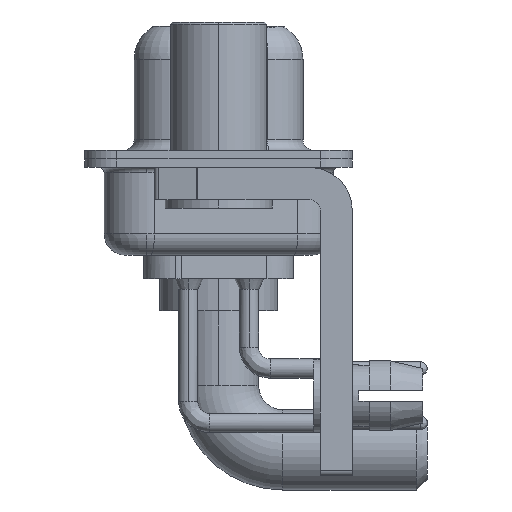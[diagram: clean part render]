
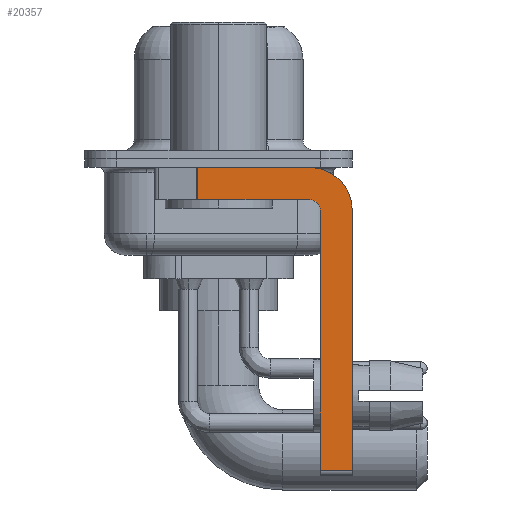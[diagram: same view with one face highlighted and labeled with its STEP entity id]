
A CAD part, left-side view. The second image highlights one B-rep face of the part: STEP entity #20357.
In plain terms, the highlighted planar face has unit normal (-1, 0, 0).
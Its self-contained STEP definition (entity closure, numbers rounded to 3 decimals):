
#67 = DIRECTION ( 'NONE',  ( 0., 1., 0. ) ) ;
#75 = CARTESIAN_POINT ( 'NONE',  ( -2.9, -4.25, -0.4 ) ) ;
#458 = EDGE_CURVE ( 'NONE', #22829, #11674, #7403, .T. ) ;
#1212 = CARTESIAN_POINT ( 'NONE',  ( -2.9, -6.25, -14.55 ) ) ;
#1302 = DIRECTION ( 'NONE',  ( 0., 0., -1. ) ) ;
#1585 = CARTESIAN_POINT ( 'NONE',  ( -2.9, -4.25, -2.4 ) ) ;
#1908 = VERTEX_POINT ( 'NONE', #1212 ) ;
#1944 = AXIS2_PLACEMENT_3D ( 'NONE', #1585, #7960, #22071 ) ;
#2185 = ORIENTED_EDGE ( 'NONE', *, *, #17712, .F. ) ;
#2240 = VERTEX_POINT ( 'NONE', #11292 ) ;
#2496 = CARTESIAN_POINT ( 'NONE',  ( -2.9, -6.25, -2.4 ) ) ;
#2915 = LINE ( 'NONE', #19490, #25348 ) ;
#3138 = VECTOR ( 'NONE', #67, 1000. ) ;
#3309 = DIRECTION ( 'NONE',  ( 0., 0., 1. ) ) ;
#4119 = CARTESIAN_POINT ( 'NONE',  ( -2.9, -4.25, -1.9 ) ) ;
#4531 = CARTESIAN_POINT ( 'NONE',  ( -2.9, -4.25, -2.4 ) ) ;
#4734 = FACE_OUTER_BOUND ( 'NONE', #25902, .T. ) ;
#5953 = ORIENTED_EDGE ( 'NONE', *, *, #12945, .T. ) ;
#6385 = VECTOR ( 'NONE', #1302, 1000. ) ;
#6635 = PLANE ( 'NONE',  #25608 ) ;
#7281 = CARTESIAN_POINT ( 'NONE',  ( -2.9, 0.978, -1.9 ) ) ;
#7403 = LINE ( 'NONE', #7281, #6385 ) ;
#7960 = DIRECTION ( 'NONE',  ( -1., 0., 0. ) ) ;
#8076 = LINE ( 'NONE', #19209, #13246 ) ;
#8776 = VERTEX_POINT ( 'NONE', #75 ) ;
#8987 = DIRECTION ( 'NONE',  ( 0., -1., 0. ) ) ;
#9568 = CARTESIAN_POINT ( 'NONE',  ( -2.9, 3., -0.4 ) ) ;
#10225 = VECTOR ( 'NONE', #20009, 1000. ) ;
#10948 = VERTEX_POINT ( 'NONE', #14437 ) ;
#11292 = CARTESIAN_POINT ( 'NONE',  ( -2.9, -4.75, -2.4 ) ) ;
#11674 = VERTEX_POINT ( 'NONE', #16979 ) ;
#11741 = LINE ( 'NONE', #9568, #10225 ) ;
#12421 = VERTEX_POINT ( 'NONE', #2496 ) ;
#12475 = CARTESIAN_POINT ( 'NONE',  ( -2.9, -4.25, -1.9 ) ) ;
#12802 = ORIENTED_EDGE ( 'NONE', *, *, #15644, .F. ) ;
#12945 = EDGE_CURVE ( 'NONE', #10948, #1908, #13219, .T. ) ;
#13051 = DIRECTION ( 'NONE',  ( 1., 0., 0. ) ) ;
#13219 = LINE ( 'NONE', #17435, #19891 ) ;
#13246 = VECTOR ( 'NONE', #24734, 1000. ) ;
#14437 = CARTESIAN_POINT ( 'NONE',  ( -2.9, -4.75, -14.55 ) ) ;
#14476 = LINE ( 'NONE', #4119, #3138 ) ;
#14824 = DIRECTION ( 'NONE',  ( 0., 0., -1. ) ) ;
#15644 = EDGE_CURVE ( 'NONE', #8776, #12421, #19301, .T. ) ;
#16699 = ORIENTED_EDGE ( 'NONE', *, *, #25475, .F. ) ;
#16734 = EDGE_CURVE ( 'NONE', #2240, #23734, #17162, .T. ) ;
#16979 = CARTESIAN_POINT ( 'NONE',  ( -2.9, 0.978, -1.9 ) ) ;
#17141 = EDGE_CURVE ( 'NONE', #10948, #2240, #2915, .T. ) ;
#17162 = CIRCLE ( 'NONE', #1944, 0.5 ) ;
#17435 = CARTESIAN_POINT ( 'NONE',  ( -2.9, -4.25, -14.55 ) ) ;
#17712 = EDGE_CURVE ( 'NONE', #22829, #8776, #11741, .T. ) ;
#18380 = AXIS2_PLACEMENT_3D ( 'NONE', #4531, #19078, #19330 ) ;
#19078 = DIRECTION ( 'NONE',  ( 1., 0., 0. ) ) ;
#19209 = CARTESIAN_POINT ( 'NONE',  ( -2.9, -6.25, -2.4 ) ) ;
#19301 = CIRCLE ( 'NONE', #18380, 2. ) ;
#19330 = DIRECTION ( 'NONE',  ( 0., 0., -1. ) ) ;
#19490 = CARTESIAN_POINT ( 'NONE',  ( -2.9, -4.75, -14.8 ) ) ;
#19891 = VECTOR ( 'NONE', #8987, 1000. ) ;
#20009 = DIRECTION ( 'NONE',  ( 0., -1., 0. ) ) ;
#20357 = ADVANCED_FACE ( 'NONE', ( #4734 ), #6635, .F. ) ;
#21530 = ORIENTED_EDGE ( 'NONE', *, *, #16734, .F. ) ;
#22055 = ORIENTED_EDGE ( 'NONE', *, *, #17141, .F. ) ;
#22071 = DIRECTION ( 'NONE',  ( 0., 0., 1. ) ) ;
#22095 = ORIENTED_EDGE ( 'NONE', *, *, #22131, .F. ) ;
#22131 = EDGE_CURVE ( 'NONE', #23734, #11674, #14476, .T. ) ;
#22774 = CARTESIAN_POINT ( 'NONE',  ( -2.9, -4.25, -2.4 ) ) ;
#22788 = ORIENTED_EDGE ( 'NONE', *, *, #458, .T. ) ;
#22829 = VERTEX_POINT ( 'NONE', #25909 ) ;
#23734 = VERTEX_POINT ( 'NONE', #12475 ) ;
#24734 = DIRECTION ( 'NONE',  ( 0., 0., -1. ) ) ;
#25348 = VECTOR ( 'NONE', #3309, 1000. ) ;
#25475 = EDGE_CURVE ( 'NONE', #12421, #1908, #8076, .T. ) ;
#25608 = AXIS2_PLACEMENT_3D ( 'NONE', #22774, #13051, #14824 ) ;
#25902 = EDGE_LOOP ( 'NONE', ( #2185, #22788, #22095, #21530, #22055, #5953, #16699, #12802 ) ) ;
#25909 = CARTESIAN_POINT ( 'NONE',  ( -2.9, 0.978, -0.4 ) ) ;
